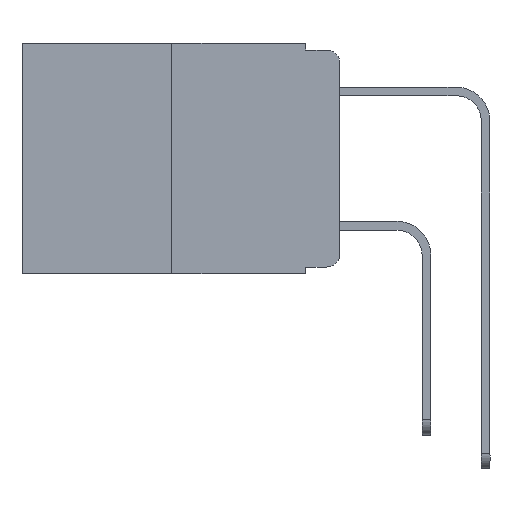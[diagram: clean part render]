
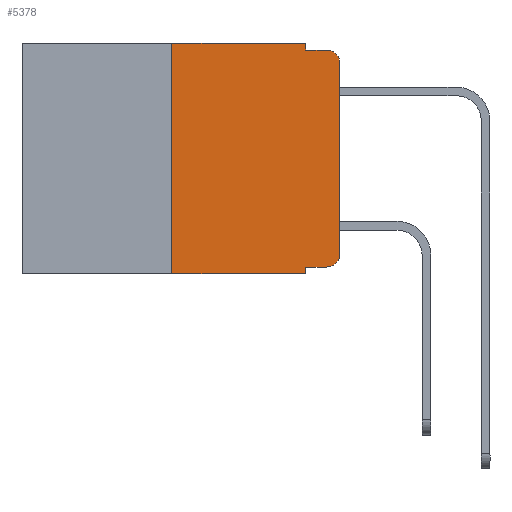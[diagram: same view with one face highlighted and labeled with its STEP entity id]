
A CAD part, left-side view. The second image highlights one B-rep face of the part: STEP entity #5378.
In plain terms, the highlighted planar face has unit normal (-1, 0, 0).
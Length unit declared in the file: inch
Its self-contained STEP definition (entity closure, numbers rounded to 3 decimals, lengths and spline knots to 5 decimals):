
#107 = LINE ( 'NONE', #5562, #9666 ) ;
#473 = VERTEX_POINT ( 'NONE', #16709 ) ;
#695 = LINE ( 'NONE', #4648, #3830 ) ;
#819 = EDGE_CURVE ( 'NONE', #16228, #9148, #14840, .T. ) ;
#1776 = ORIENTED_EDGE ( 'NONE', *, *, #14750, .T. ) ;
#2258 = DIRECTION ( 'NONE',  ( 0., 0., 1. ) ) ;
#2447 = CARTESIAN_POINT ( 'NONE',  ( 0., 0.473, 0. ) ) ;
#2829 = DIRECTION ( 'NONE',  ( 0., -1., 0. ) ) ;
#3001 = ORIENTED_EDGE ( 'NONE', *, *, #17028, .T. ) ;
#3542 = DIRECTION ( 'NONE',  ( 0., 0., -1. ) ) ;
#3563 = EDGE_CURVE ( 'NONE', #17186, #7544, #11120, .T. ) ;
#3777 = PLANE ( 'NONE',  #14233 ) ;
#3789 = ORIENTED_EDGE ( 'NONE', *, *, #9674, .F. ) ;
#3830 = VECTOR ( 'NONE', #5692, 39.37008 ) ;
#4242 = DIRECTION ( 'NONE',  ( 0., 0., 1. ) ) ;
#4363 = CARTESIAN_POINT ( 'NONE',  ( 0., 0.02, -0.333 ) ) ;
#4405 = VERTEX_POINT ( 'NONE', #12125 ) ;
#4581 = VECTOR ( 'NONE', #14826, 39.37008 ) ;
#4648 = CARTESIAN_POINT ( 'NONE',  ( 0., 0.051, 0. ) ) ;
#4768 = DIRECTION ( 'NONE',  ( -1., 0., 0. ) ) ;
#5165 = AXIS2_PLACEMENT_3D ( 'NONE', #15229, #15728, #16635 ) ;
#5378 = ADVANCED_FACE ( 'NONE', ( #9277 ), #3777, .F. ) ;
#5562 = CARTESIAN_POINT ( 'NONE',  ( 0., 0.473, 0. ) ) ;
#5692 = DIRECTION ( 'NONE',  ( 0., 0., -1. ) ) ;
#6079 = AXIS2_PLACEMENT_3D ( 'NONE', #9927, #4768, #3542 ) ;
#6551 = CARTESIAN_POINT ( 'NONE',  ( 0., 0.051, 0. ) ) ;
#6642 = ORIENTED_EDGE ( 'NONE', *, *, #12616, .F. ) ;
#6820 = CARTESIAN_POINT ( 'NONE',  ( 0., 0.473, -0.343 ) ) ;
#6935 = CARTESIAN_POINT ( 'NONE',  ( 0., 0.051, -0.333 ) ) ;
#7212 = CARTESIAN_POINT ( 'NONE',  ( 0., 0.051, 0. ) ) ;
#7247 = ORIENTED_EDGE ( 'NONE', *, *, #3563, .T. ) ;
#7303 = CARTESIAN_POINT ( 'NONE',  ( 0., 0., -0.03 ) ) ;
#7544 = VERTEX_POINT ( 'NONE', #10645 ) ;
#7646 = CARTESIAN_POINT ( 'NONE',  ( 0., 0.051, -0.01 ) ) ;
#7837 = VERTEX_POINT ( 'NONE', #10906 ) ;
#8346 = EDGE_LOOP ( 'NONE', ( #3001, #7247, #3789, #14539, #9790, #16498, #1776, #6642, #12114, #15443 ) ) ;
#8701 = EDGE_CURVE ( 'NONE', #16412, #7837, #695, .T. ) ;
#8934 = VERTEX_POINT ( 'NONE', #13067 ) ;
#9033 = DIRECTION ( 'NONE',  ( 0., -1., 0. ) ) ;
#9148 = VERTEX_POINT ( 'NONE', #4363 ) ;
#9277 = FACE_OUTER_BOUND ( 'NONE', #8346, .T. ) ;
#9491 = CARTESIAN_POINT ( 'NONE',  ( 0., 0., 0. ) ) ;
#9629 = CIRCLE ( 'NONE', #5165, 0.02 ) ;
#9666 = VECTOR ( 'NONE', #2829, 39.37008 ) ;
#9674 = EDGE_CURVE ( 'NONE', #7837, #7544, #10434, .T. ) ;
#9790 = ORIENTED_EDGE ( 'NONE', *, *, #17022, .F. ) ;
#9927 = CARTESIAN_POINT ( 'NONE',  ( 0., 0.02, -0.03 ) ) ;
#10434 = LINE ( 'NONE', #7646, #13106 ) ;
#10645 = CARTESIAN_POINT ( 'NONE',  ( 0., 0.02, -0.01 ) ) ;
#10906 = CARTESIAN_POINT ( 'NONE',  ( 0., 0.051, -0.01 ) ) ;
#11009 = EDGE_CURVE ( 'NONE', #9148, #14194, #9629, .T. ) ;
#11036 = DIRECTION ( 'NONE',  ( 0., -1., 0. ) ) ;
#11120 = CIRCLE ( 'NONE', #6079, 0.02 ) ;
#11490 = EDGE_CURVE ( 'NONE', #4405, #8934, #14301, .T. ) ;
#11762 = CARTESIAN_POINT ( 'NONE',  ( 0., 0., -0.313 ) ) ;
#11829 = DIRECTION ( 'NONE',  ( 0., 0., -1. ) ) ;
#12000 = LINE ( 'NONE', #6820, #4581 ) ;
#12114 = ORIENTED_EDGE ( 'NONE', *, *, #819, .T. ) ;
#12125 = CARTESIAN_POINT ( 'NONE',  ( 0., 0.25, -0.343 ) ) ;
#12616 = EDGE_CURVE ( 'NONE', #16228, #473, #15125, .T. ) ;
#13067 = CARTESIAN_POINT ( 'NONE',  ( 0., 0.25, 0. ) ) ;
#13106 = VECTOR ( 'NONE', #9033, 39.37008 ) ;
#13161 = DIRECTION ( 'NONE',  ( 1., 0., 0. ) ) ;
#13217 = VECTOR ( 'NONE', #2258, 39.37008 ) ;
#14066 = DIRECTION ( 'NONE',  ( 0., 0., -1. ) ) ;
#14190 = VECTOR ( 'NONE', #4242, 39.37008 ) ;
#14194 = VERTEX_POINT ( 'NONE', #11762 ) ;
#14233 = AXIS2_PLACEMENT_3D ( 'NONE', #2447, #13161, #11829 ) ;
#14295 = CARTESIAN_POINT ( 'NONE',  ( 0., 0.051, -0.333 ) ) ;
#14301 = LINE ( 'NONE', #16768, #13217 ) ;
#14539 = ORIENTED_EDGE ( 'NONE', *, *, #8701, .F. ) ;
#14750 = EDGE_CURVE ( 'NONE', #4405, #473, #12000, .T. ) ;
#14826 = DIRECTION ( 'NONE',  ( 0., -1., 0. ) ) ;
#14840 = LINE ( 'NONE', #6935, #16187 ) ;
#15125 = LINE ( 'NONE', #7212, #16303 ) ;
#15229 = CARTESIAN_POINT ( 'NONE',  ( 0., 0.02, -0.313 ) ) ;
#15443 = ORIENTED_EDGE ( 'NONE', *, *, #11009, .T. ) ;
#15728 = DIRECTION ( 'NONE',  ( -1., 0., 0. ) ) ;
#16187 = VECTOR ( 'NONE', #11036, 39.37008 ) ;
#16228 = VERTEX_POINT ( 'NONE', #14295 ) ;
#16286 = LINE ( 'NONE', #9491, #14190 ) ;
#16303 = VECTOR ( 'NONE', #14066, 39.37008 ) ;
#16412 = VERTEX_POINT ( 'NONE', #6551 ) ;
#16498 = ORIENTED_EDGE ( 'NONE', *, *, #11490, .F. ) ;
#16635 = DIRECTION ( 'NONE',  ( 0., 0., -1. ) ) ;
#16709 = CARTESIAN_POINT ( 'NONE',  ( 0., 0.051, -0.343 ) ) ;
#16768 = CARTESIAN_POINT ( 'NONE',  ( 0., 0.25, 0. ) ) ;
#17022 = EDGE_CURVE ( 'NONE', #8934, #16412, #107, .T. ) ;
#17028 = EDGE_CURVE ( 'NONE', #14194, #17186, #16286, .T. ) ;
#17186 = VERTEX_POINT ( 'NONE', #7303 ) ;
